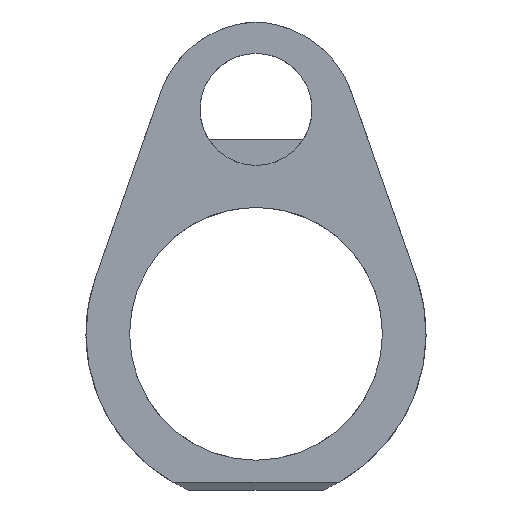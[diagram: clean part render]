
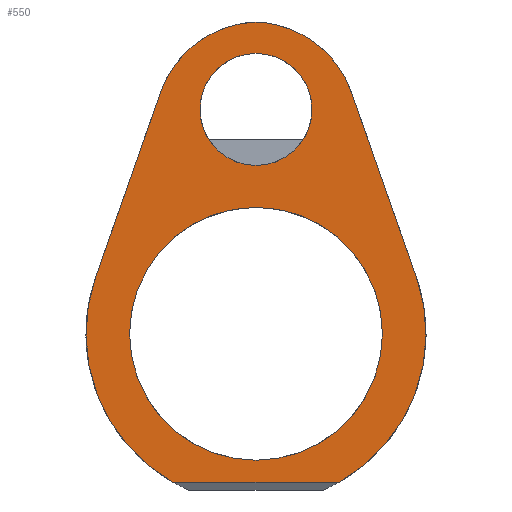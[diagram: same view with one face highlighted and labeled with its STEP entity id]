
A CAD part, left-side view. The second image highlights one B-rep face of the part: STEP entity #550.
In plain terms, the highlighted planar face has unit normal (-1, 0, 0).
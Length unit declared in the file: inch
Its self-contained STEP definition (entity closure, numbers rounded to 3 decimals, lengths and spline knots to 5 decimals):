
#34=PLANE('',#619);
#41=FACE_BOUND('',#107,.T.);
#42=FACE_BOUND('',#108,.T.);
#71=FACE_OUTER_BOUND('',#106,.T.);
#106=EDGE_LOOP('',(#500,#501,#502,#503,#504,#505,#506));
#107=EDGE_LOOP('',(#507));
#108=EDGE_LOOP('',(#508));
#118=B_SPLINE_CURVE_WITH_KNOTS('',3,(#1070,#1071,#1072,#1073,#1074,#1075,
#1076,#1077,#1078,#1079,#1080,#1081,#1082,#1083),.UNSPECIFIED.,.F.,.F.,
(4,2,2,2,2,2,4),(0.19727,0.20591,0.57332,
0.80296,1.03279,1.40053,1.60717),
 .UNSPECIFIED.);
#119=B_SPLINE_CURVE_WITH_KNOTS('',3,(#1114,#1115,#1116,#1117,#1118,#1119,
#1120,#1121,#1122,#1123,#1124,#1125,#1126,#1127),.UNSPECIFIED.,.F.,.F.,
(4,2,2,2,2,2,4),(0.04445,0.25108,0.61882,
0.84866,1.07829,1.44571,1.45435),
 .UNSPECIFIED.);
#138=LINE('',#951,#177);
#147=LINE('',#976,#186);
#155=LINE('',#1032,#194);
#177=VECTOR('',#704,0.3937);
#186=VECTOR('',#731,0.3937);
#194=VECTOR('',#761,0.3937);
#198=CIRCLE('',#566,0.5635);
#212=CIRCLE('',#598,0.7579);
#215=CIRCLE('',#602,0.7579);
#221=CIRCLE('',#618,0.2495);
#222=VERTEX_POINT('',#773);
#254=VERTEX_POINT('',#945);
#256=VERTEX_POINT('',#949);
#257=VERTEX_POINT('',#953);
#260=VERTEX_POINT('',#963);
#263=VERTEX_POINT('',#974);
#272=VERTEX_POINT('',#1031);
#273=VERTEX_POINT('',#1035);
#274=VERTEX_POINT('',#1068);
#275=EDGE_CURVE('',#222,#222,#198,.F.);
#318=EDGE_CURVE('',#254,#256,#138,.T.);
#319=EDGE_CURVE('',#257,#254,#212,.T.);
#326=EDGE_CURVE('',#256,#260,#215,.T.);
#331=EDGE_CURVE('',#260,#263,#147,.T.);
#346=EDGE_CURVE('',#272,#257,#155,.T.);
#348=EDGE_CURVE('',#273,#273,#221,.T.);
#351=EDGE_CURVE('',#263,#274,#118,.T.);
#352=EDGE_CURVE('',#274,#272,#119,.T.);
#500=ORIENTED_EDGE('',*,*,#318,.T.);
#501=ORIENTED_EDGE('',*,*,#326,.T.);
#502=ORIENTED_EDGE('',*,*,#331,.T.);
#503=ORIENTED_EDGE('',*,*,#351,.T.);
#504=ORIENTED_EDGE('',*,*,#352,.T.);
#505=ORIENTED_EDGE('',*,*,#346,.T.);
#506=ORIENTED_EDGE('',*,*,#319,.T.);
#507=ORIENTED_EDGE('',*,*,#275,.T.);
#508=ORIENTED_EDGE('',*,*,#348,.T.);
#550=ADVANCED_FACE('',(#71,#41,#42),#34,.F.);
#566=AXIS2_PLACEMENT_3D('',#774,#624,#625);
#598=AXIS2_PLACEMENT_3D('',#954,#707,#708);
#602=AXIS2_PLACEMENT_3D('',#965,#719,#720);
#618=AXIS2_PLACEMENT_3D('',#1036,#765,#766);
#619=AXIS2_PLACEMENT_3D('',#1128,#769,#770);
#624=DIRECTION('center_axis',(-1.,0.,0.));
#625=DIRECTION('ref_axis',(0.,-1.,0.));
#704=DIRECTION('',(0.,-1.,0.));
#707=DIRECTION('center_axis',(-1.,0.,0.));
#708=DIRECTION('ref_axis',(0.,0.941,0.339));
#719=DIRECTION('center_axis',(-1.,0.,0.));
#720=DIRECTION('ref_axis',(0.,-0.396,-0.918));
#731=DIRECTION('',(0.,0.331,0.943));
#761=DIRECTION('',(0.,0.331,-0.943));
#765=DIRECTION('center_axis',(1.,0.,0.));
#766=DIRECTION('ref_axis',(0.,0.,-1.));
#769=DIRECTION('center_axis',(1.,0.,0.));
#770=DIRECTION('ref_axis',(0.,0.,
-1.));
#773=CARTESIAN_POINT('',(-2.3,0.5645,-3.2165));
#774=CARTESIAN_POINT('Origin',(-2.3,0.001,-3.2165));
#945=CARTESIAN_POINT('',(-2.3,0.3718,-3.8775));
#949=CARTESIAN_POINT('',(-2.3,-0.3698,-3.8775));
#951=CARTESIAN_POINT('',(-2.3,0.0005,-3.8775));
#953=CARTESIAN_POINT('',(-2.3,0.71607,-2.96533));
#954=CARTESIAN_POINT('Origin',(-2.3,0.001,-3.2165));
#963=CARTESIAN_POINT('',(-2.3,-0.71407,-2.96533));
#965=CARTESIAN_POINT('Origin',(-2.3,0.001,-3.2165));
#974=CARTESIAN_POINT('',(-2.3,-0.4243,-2.14035));
#976=CARTESIAN_POINT('',(-2.3,-0.71407,-2.96533));
#1031=CARTESIAN_POINT('',(-2.3,0.4263,-2.14035));
#1032=CARTESIAN_POINT('',(-2.3,0.4263,-2.14035));
#1035=CARTESIAN_POINT('',(-2.3,0.001,-1.967));
#1036=CARTESIAN_POINT('Origin',(-2.3,0.001,-2.2165));
#1068=CARTESIAN_POINT('',(-2.3,0.001,-1.82686));
#1070=CARTESIAN_POINT('Ctrl Pts',(-2.3,-0.4243,-2.14035));
#1071=CARTESIAN_POINT('Ctrl Pts',(-2.3,-0.42392,-2.13927));
#1072=CARTESIAN_POINT('Ctrl Pts',(-2.3,-0.42354,-2.13819));
#1073=CARTESIAN_POINT('Ctrl Pts',(-2.3,-0.40666,-2.09125));
#1074=CARTESIAN_POINT('Ctrl Pts',(-2.3,-0.38296,-2.04799));
#1075=CARTESIAN_POINT('Ctrl Pts',(-2.3,-0.33456,-1.98529));
#1076=CARTESIAN_POINT('Ctrl Pts',(-2.3,-0.31359,-1.96299));
#1077=CARTESIAN_POINT('Ctrl Pts',(-2.3,-0.26772,-1.92287));
#1078=CARTESIAN_POINT('Ctrl Pts',(-2.3,-0.24281,-1.90504));
#1079=CARTESIAN_POINT('Ctrl Pts',(-2.3,-0.17418,-1.86537));
#1080=CARTESIAN_POINT('Ctrl Pts',(-2.3,-0.12813,-1.84758));
#1081=CARTESIAN_POINT('Ctrl Pts',(-2.3,-0.05368,-1.83142));
#1082=CARTESIAN_POINT('Ctrl Pts',(-2.3,-0.02639,-1.82795));
#1083=CARTESIAN_POINT('Ctrl Pts',(-2.3,0.001,-1.82686));
#1114=CARTESIAN_POINT('Ctrl Pts',(-2.3,0.001,-1.82686));
#1115=CARTESIAN_POINT('Ctrl Pts',(-2.3,0.02839,-1.82795));
#1116=CARTESIAN_POINT('Ctrl Pts',(-2.3,0.05568,-1.83142));
#1117=CARTESIAN_POINT('Ctrl Pts',(-2.3,0.13013,-1.84758));
#1118=CARTESIAN_POINT('Ctrl Pts',(-2.3,0.17618,-1.86537));
#1119=CARTESIAN_POINT('Ctrl Pts',(-2.3,0.24481,-1.90504));
#1120=CARTESIAN_POINT('Ctrl Pts',(-2.3,0.26972,-1.92287));
#1121=CARTESIAN_POINT('Ctrl Pts',(-2.3,0.31559,-1.96299));
#1122=CARTESIAN_POINT('Ctrl Pts',(-2.3,0.33656,-1.98529));
#1123=CARTESIAN_POINT('Ctrl Pts',(-2.3,0.38496,-2.04799));
#1124=CARTESIAN_POINT('Ctrl Pts',(-2.3,0.40866,-2.09125));
#1125=CARTESIAN_POINT('Ctrl Pts',(-2.3,0.42554,-2.13819));
#1126=CARTESIAN_POINT('Ctrl Pts',(-2.3,0.42592,-2.13927));
#1127=CARTESIAN_POINT('Ctrl Pts',(-2.3,0.4263,-2.14035));
#1128=CARTESIAN_POINT('Origin',(-2.3,0.001,-2.94183));
